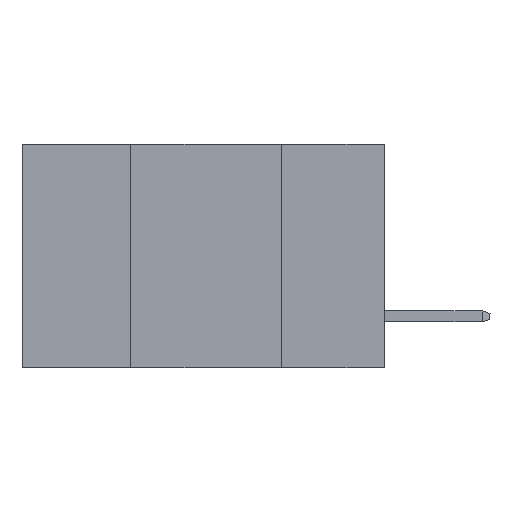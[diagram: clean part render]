
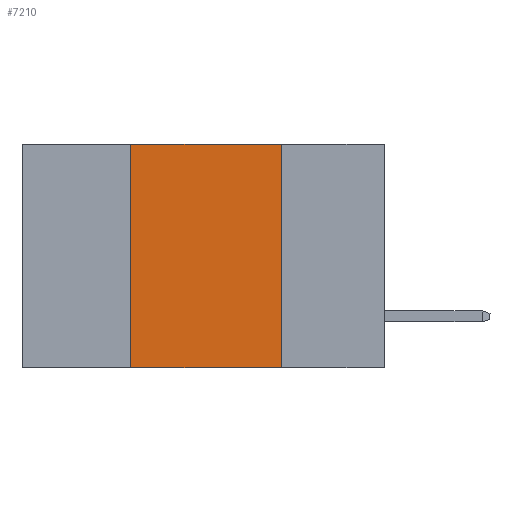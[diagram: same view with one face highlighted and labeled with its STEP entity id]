
A CAD part, left-side view. The second image highlights one B-rep face of the part: STEP entity #7210.
In plain terms, the highlighted planar face has unit normal (-1, 0, 0).
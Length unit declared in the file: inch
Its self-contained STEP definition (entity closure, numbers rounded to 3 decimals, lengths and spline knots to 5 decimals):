
#537 = LINE ( 'NONE', #1699, #6727 ) ;
#628 = CARTESIAN_POINT ( 'NONE',  ( 0., 0.6, 0. ) ) ;
#696 = EDGE_CURVE ( 'NONE', #6352, #7144, #748, .T. ) ;
#748 = LINE ( 'NONE', #5978, #2848 ) ;
#808 = VECTOR ( 'NONE', #8539, 39.37008 ) ;
#1041 = CARTESIAN_POINT ( 'NONE',  ( 0., 0.42, 0. ) ) ;
#1341 = ORIENTED_EDGE ( 'NONE', *, *, #3643, .F. ) ;
#1491 = ORIENTED_EDGE ( 'NONE', *, *, #7610, .F. ) ;
#1699 = CARTESIAN_POINT ( 'NONE',  ( 0., 0.17, -0.37 ) ) ;
#1733 = EDGE_LOOP ( 'NONE', ( #1341, #1491, #2379, #2109 ) ) ;
#2109 = ORIENTED_EDGE ( 'NONE', *, *, #5211, .T. ) ;
#2379 = ORIENTED_EDGE ( 'NONE', *, *, #696, .F. ) ;
#2706 = CARTESIAN_POINT ( 'NONE',  ( 0., 0.17, -0.37 ) ) ;
#2848 = VECTOR ( 'NONE', #3879, 39.37008 ) ;
#3162 = CARTESIAN_POINT ( 'NONE',  ( 0., 0.17, 0. ) ) ;
#3262 = LINE ( 'NONE', #3346, #808 ) ;
#3346 = CARTESIAN_POINT ( 'NONE',  ( 0., 0.6, -0.37 ) ) ;
#3643 = EDGE_CURVE ( 'NONE', #7093, #6202, #537, .T. ) ;
#3738 = AXIS2_PLACEMENT_3D ( 'NONE', #6594, #5279, #6553 ) ;
#3755 = CARTESIAN_POINT ( 'NONE',  ( 0., 0.42, -0.37 ) ) ;
#3879 = DIRECTION ( 'NONE',  ( 0., 0., 1. ) ) ;
#4309 = DIRECTION ( 'NONE',  ( 0., 0., -1. ) ) ;
#4575 = LINE ( 'NONE', #628, #8141 ) ;
#4613 = DIRECTION ( 'NONE',  ( 0., -1., 0. ) ) ;
#4658 = FACE_OUTER_BOUND ( 'NONE', #1733, .T. ) ;
#5211 = EDGE_CURVE ( 'NONE', #6352, #6202, #3262, .T. ) ;
#5279 = DIRECTION ( 'NONE',  ( 1., 0., 0. ) ) ;
#5978 = CARTESIAN_POINT ( 'NONE',  ( 0., 0.42, -0.37 ) ) ;
#6202 = VERTEX_POINT ( 'NONE', #2706 ) ;
#6352 = VERTEX_POINT ( 'NONE', #3755 ) ;
#6553 = DIRECTION ( 'NONE',  ( 0., 0., -1. ) ) ;
#6594 = CARTESIAN_POINT ( 'NONE',  ( 0., 0.6, 0. ) ) ;
#6727 = VECTOR ( 'NONE', #4309, 39.37008 ) ;
#7093 = VERTEX_POINT ( 'NONE', #3162 ) ;
#7144 = VERTEX_POINT ( 'NONE', #1041 ) ;
#7208 = PLANE ( 'NONE',  #3738 ) ;
#7210 = ADVANCED_FACE ( 'NONE', ( #4658 ), #7208, .F. ) ;
#7610 = EDGE_CURVE ( 'NONE', #7144, #7093, #4575, .T. ) ;
#8141 = VECTOR ( 'NONE', #4613, 39.37008 ) ;
#8539 = DIRECTION ( 'NONE',  ( 0., -1., 0. ) ) ;
